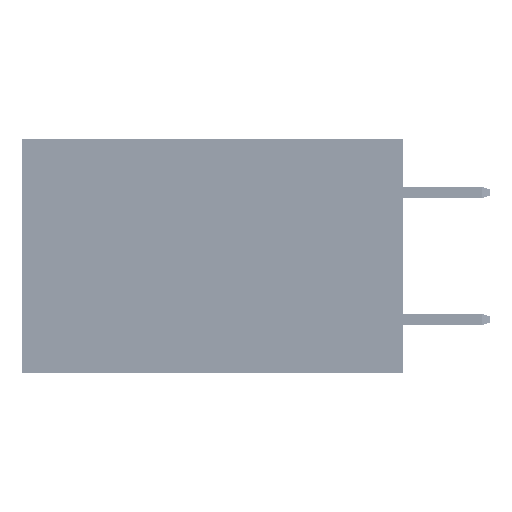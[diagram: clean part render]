
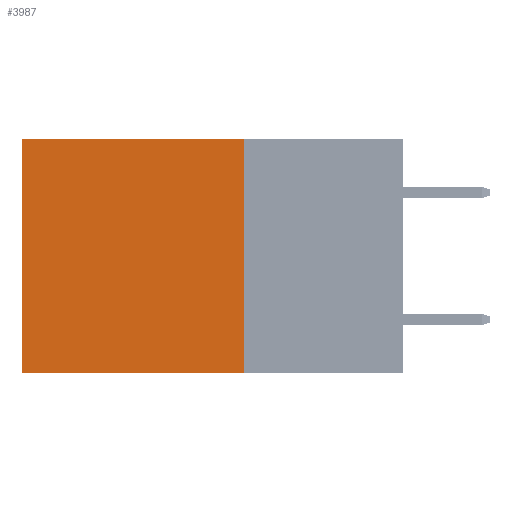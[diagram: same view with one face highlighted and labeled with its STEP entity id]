
A CAD part, left-side view. The second image highlights one B-rep face of the part: STEP entity #3987.
In plain terms, the highlighted planar face has unit normal (-1, 0, 0).
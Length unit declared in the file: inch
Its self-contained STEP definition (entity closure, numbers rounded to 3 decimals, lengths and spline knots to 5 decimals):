
#97 = DIRECTION ( 'NONE',  ( 0., 1., 0. ) ) ;
#247 = ORIENTED_EDGE ( 'NONE', *, *, #3845, .F. ) ;
#1565 = LINE ( 'NONE', #41696, #37247 ) ;
#3757 = CARTESIAN_POINT ( 'NONE',  ( 0.2875, 0.25, -0.37 ) ) ;
#3845 = EDGE_CURVE ( 'NONE', #5980, #10382, #30292, .T. ) ;
#3987 = ADVANCED_FACE ( 'NONE', ( #34643 ), #24451, .F. ) ;
#4836 = VECTOR ( 'NONE', #97, 39.37008 ) ;
#5253 = DIRECTION ( 'NONE',  ( 1., 0., 0. ) ) ;
#5980 = VERTEX_POINT ( 'NONE', #10049 ) ;
#7467 = EDGE_LOOP ( 'NONE', ( #44518, #23515, #247, #19233 ) ) ;
#7917 = VECTOR ( 'NONE', #18569, 39.37008 ) ;
#10049 = CARTESIAN_POINT ( 'NONE',  ( 0.2875, 0.25, 0. ) ) ;
#10382 = VERTEX_POINT ( 'NONE', #22539 ) ;
#11466 = VERTEX_POINT ( 'NONE', #45692 ) ;
#12133 = EDGE_CURVE ( 'NONE', #5980, #14436, #33383, .T. ) ;
#14032 = CARTESIAN_POINT ( 'NONE',  ( 0.2875, 0.6, 0. ) ) ;
#14436 = VERTEX_POINT ( 'NONE', #14032 ) ;
#18314 = CARTESIAN_POINT ( 'NONE',  ( 0.2875, 0.25, 0. ) ) ;
#18569 = DIRECTION ( 'NONE',  ( 0., 1., 0. ) ) ;
#19233 = ORIENTED_EDGE ( 'NONE', *, *, #12133, .T. ) ;
#22202 = AXIS2_PLACEMENT_3D ( 'NONE', #39024, #5253, #31711 ) ;
#22539 = CARTESIAN_POINT ( 'NONE',  ( 0.2875, 0.25, -0.37 ) ) ;
#23515 = ORIENTED_EDGE ( 'NONE', *, *, #26028, .F. ) ;
#23770 = VECTOR ( 'NONE', #40764, 39.37008 ) ;
#24451 = PLANE ( 'NONE',  #22202 ) ;
#26028 = EDGE_CURVE ( 'NONE', #10382, #11466, #26347, .T. ) ;
#26347 = LINE ( 'NONE', #3757, #7917 ) ;
#30292 = LINE ( 'NONE', #33940, #23770 ) ;
#31711 = DIRECTION ( 'NONE',  ( 0., 0., -1. ) ) ;
#33383 = LINE ( 'NONE', #18314, #4836 ) ;
#33940 = CARTESIAN_POINT ( 'NONE',  ( 0.2875, 0.25, 0. ) ) ;
#34403 = EDGE_CURVE ( 'NONE', #14436, #11466, #1565, .T. ) ;
#34643 = FACE_OUTER_BOUND ( 'NONE', #7467, .T. ) ;
#37247 = VECTOR ( 'NONE', #42647, 39.37008 ) ;
#39024 = CARTESIAN_POINT ( 'NONE',  ( 0.2875, 0.25, 0. ) ) ;
#40764 = DIRECTION ( 'NONE',  ( 0., 0., -1. ) ) ;
#41696 = CARTESIAN_POINT ( 'NONE',  ( 0.2875, 0.6, 0. ) ) ;
#42647 = DIRECTION ( 'NONE',  ( 0., 0., -1. ) ) ;
#44518 = ORIENTED_EDGE ( 'NONE', *, *, #34403, .T. ) ;
#45692 = CARTESIAN_POINT ( 'NONE',  ( 0.2875, 0.6, -0.37 ) ) ;
